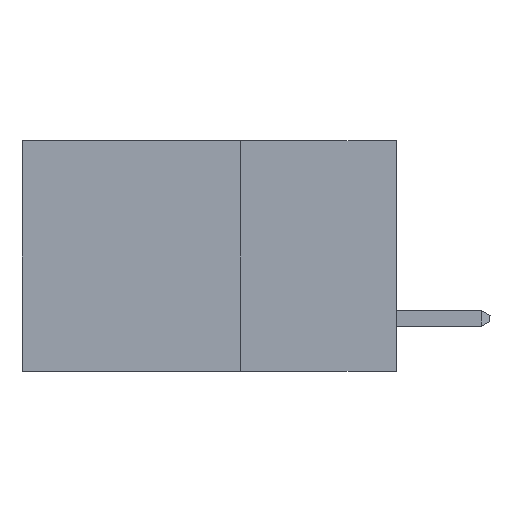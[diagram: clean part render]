
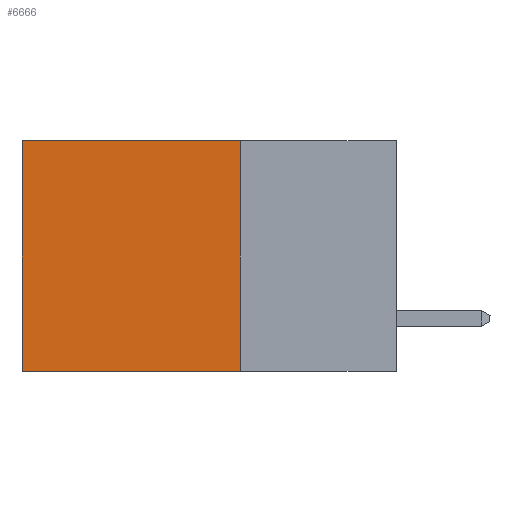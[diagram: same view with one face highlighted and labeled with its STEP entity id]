
A CAD part, left-side view. The second image highlights one B-rep face of the part: STEP entity #6666.
In plain terms, the highlighted planar face has unit normal (-1, 0, 0).
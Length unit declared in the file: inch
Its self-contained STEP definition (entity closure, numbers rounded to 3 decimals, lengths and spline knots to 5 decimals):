
#793 = CARTESIAN_POINT ( 'NONE',  ( 0.2615, 0.6, -0.37 ) ) ;
#834 = ORIENTED_EDGE ( 'NONE', *, *, #17702, .T. ) ;
#1198 = EDGE_CURVE ( 'NONE', #2854, #16586, #8078, .T. ) ;
#1936 = VECTOR ( 'NONE', #9893, 39.37008 ) ;
#2854 = VERTEX_POINT ( 'NONE', #4959 ) ;
#3053 = EDGE_LOOP ( 'NONE', ( #4927, #16931, #13364, #834 ) ) ;
#3528 = FACE_OUTER_BOUND ( 'NONE', #3053, .T. ) ;
#4000 = CARTESIAN_POINT ( 'NONE',  ( 0.2615, 0.25, 0. ) ) ;
#4187 = VECTOR ( 'NONE', #13004, 39.37008 ) ;
#4425 = EDGE_CURVE ( 'NONE', #6650, #17925, #13573, .T. ) ;
#4507 = CARTESIAN_POINT ( 'NONE',  ( 0.2615, 0.25, -0.37 ) ) ;
#4927 = ORIENTED_EDGE ( 'NONE', *, *, #1198, .T. ) ;
#4959 = CARTESIAN_POINT ( 'NONE',  ( 0.2615, 0.6, 0. ) ) ;
#5692 = DIRECTION ( 'NONE',  ( 0., 0., -1. ) ) ;
#5753 = DIRECTION ( 'NONE',  ( 1., 0., 0. ) ) ;
#5789 = CARTESIAN_POINT ( 'NONE',  ( 0.2615, 0.25, -0.37 ) ) ;
#6151 = PLANE ( 'NONE',  #7440 ) ;
#6650 = VERTEX_POINT ( 'NONE', #6738 ) ;
#6666 = ADVANCED_FACE ( 'NONE', ( #3528 ), #6151, .F. ) ;
#6738 = CARTESIAN_POINT ( 'NONE',  ( 0.2615, 0.25, 0. ) ) ;
#7440 = AXIS2_PLACEMENT_3D ( 'NONE', #5789, #5753, #5692 ) ;
#7523 = VECTOR ( 'NONE', #15479, 39.37008 ) ;
#8078 = LINE ( 'NONE', #15915, #4187 ) ;
#9893 = DIRECTION ( 'NONE',  ( 0., 0., -1. ) ) ;
#10187 = CARTESIAN_POINT ( 'NONE',  ( 0.2615, 0.25, -0.37 ) ) ;
#12087 = VECTOR ( 'NONE', #15818, 39.37008 ) ;
#13004 = DIRECTION ( 'NONE',  ( 0., 0., -1. ) ) ;
#13364 = ORIENTED_EDGE ( 'NONE', *, *, #4425, .F. ) ;
#13573 = LINE ( 'NONE', #10187, #1936 ) ;
#14442 = CARTESIAN_POINT ( 'NONE',  ( 0.2615, 0.25, -0.37 ) ) ;
#15479 = DIRECTION ( 'NONE',  ( 0., 1., 0. ) ) ;
#15818 = DIRECTION ( 'NONE',  ( 0., 1., 0. ) ) ;
#15915 = CARTESIAN_POINT ( 'NONE',  ( 0.2615, 0.6, -0.37 ) ) ;
#15999 = LINE ( 'NONE', #4000, #7523 ) ;
#16205 = LINE ( 'NONE', #14442, #12087 ) ;
#16586 = VERTEX_POINT ( 'NONE', #793 ) ;
#16931 = ORIENTED_EDGE ( 'NONE', *, *, #17861, .F. ) ;
#17702 = EDGE_CURVE ( 'NONE', #6650, #2854, #15999, .T. ) ;
#17861 = EDGE_CURVE ( 'NONE', #17925, #16586, #16205, .T. ) ;
#17925 = VERTEX_POINT ( 'NONE', #4507 ) ;
